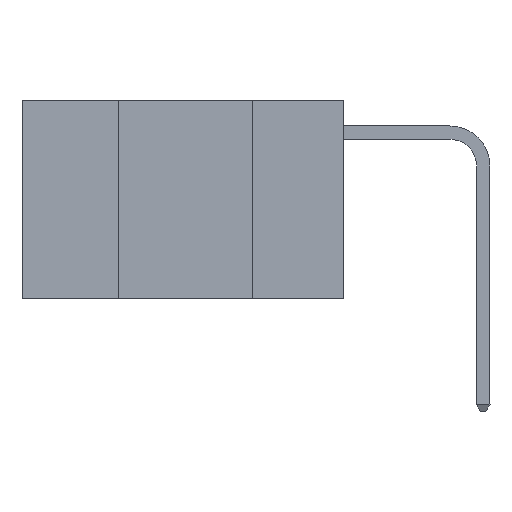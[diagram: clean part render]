
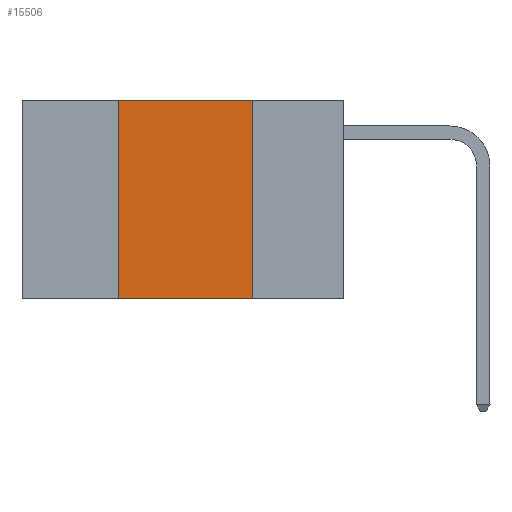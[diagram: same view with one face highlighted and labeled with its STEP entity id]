
A CAD part, left-side view. The second image highlights one B-rep face of the part: STEP entity #15506.
In plain terms, the highlighted planar face has unit normal (-1, 0, 0).
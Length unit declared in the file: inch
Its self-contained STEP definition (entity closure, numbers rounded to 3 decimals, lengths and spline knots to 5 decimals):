
#364 = PLANE ( 'NONE',  #12831 ) ;
#907 = VERTEX_POINT ( 'NONE', #16280 ) ;
#945 = DIRECTION ( 'NONE',  ( 0., 0., 1. ) ) ;
#2093 = DIRECTION ( 'NONE',  ( 0., 0., -1. ) ) ;
#3798 = CARTESIAN_POINT ( 'NONE',  ( 0., 0.6, -0.37 ) ) ;
#4659 = VERTEX_POINT ( 'NONE', #12384 ) ;
#5478 = CARTESIAN_POINT ( 'NONE',  ( 0., 0.6, 0. ) ) ;
#6419 = CARTESIAN_POINT ( 'NONE',  ( 0., 0.17, 0. ) ) ;
#6572 = DIRECTION ( 'NONE',  ( 0., -1., 0. ) ) ;
#7718 = CARTESIAN_POINT ( 'NONE',  ( 0., 0.42, 0. ) ) ;
#7803 = EDGE_CURVE ( 'NONE', #16670, #907, #17395, .T. ) ;
#8090 = DIRECTION ( 'NONE',  ( 0., 0., -1. ) ) ;
#8776 = LINE ( 'NONE', #16272, #12580 ) ;
#8827 = VECTOR ( 'NONE', #8090, 39.37008 ) ;
#9181 = EDGE_CURVE ( 'NONE', #16499, #16670, #8776, .T. ) ;
#10341 = CARTESIAN_POINT ( 'NONE',  ( 0., 0.17, 0. ) ) ;
#11223 = VECTOR ( 'NONE', #13628, 39.37008 ) ;
#12099 = DIRECTION ( 'NONE',  ( 1., 0., 0. ) ) ;
#12356 = ORIENTED_EDGE ( 'NONE', *, *, #7803, .F. ) ;
#12384 = CARTESIAN_POINT ( 'NONE',  ( 0., 0.42, -0.37 ) ) ;
#12562 = ORIENTED_EDGE ( 'NONE', *, *, #9181, .F. ) ;
#12578 = ORIENTED_EDGE ( 'NONE', *, *, #17608, .F. ) ;
#12580 = VECTOR ( 'NONE', #6572, 39.37008 ) ;
#12723 = ORIENTED_EDGE ( 'NONE', *, *, #14879, .T. ) ;
#12831 = AXIS2_PLACEMENT_3D ( 'NONE', #5478, #12099, #2093 ) ;
#13532 = VECTOR ( 'NONE', #945, 39.37008 ) ;
#13628 = DIRECTION ( 'NONE',  ( 0., -1., 0. ) ) ;
#14772 = CARTESIAN_POINT ( 'NONE',  ( 0., 0.42, 0. ) ) ;
#14879 = EDGE_CURVE ( 'NONE', #4659, #907, #19692, .T. ) ;
#15426 = EDGE_LOOP ( 'NONE', ( #12356, #12562, #12578, #12723 ) ) ;
#15506 = ADVANCED_FACE ( 'NONE', ( #19422 ), #364, .F. ) ;
#16272 = CARTESIAN_POINT ( 'NONE',  ( 0., 0.6, 0. ) ) ;
#16280 = CARTESIAN_POINT ( 'NONE',  ( 0., 0.17, -0.37 ) ) ;
#16499 = VERTEX_POINT ( 'NONE', #14772 ) ;
#16670 = VERTEX_POINT ( 'NONE', #10341 ) ;
#17395 = LINE ( 'NONE', #6419, #8827 ) ;
#17608 = EDGE_CURVE ( 'NONE', #4659, #16499, #17806, .T. ) ;
#17806 = LINE ( 'NONE', #7718, #13532 ) ;
#19422 = FACE_OUTER_BOUND ( 'NONE', #15426, .T. ) ;
#19692 = LINE ( 'NONE', #3798, #11223 ) ;
